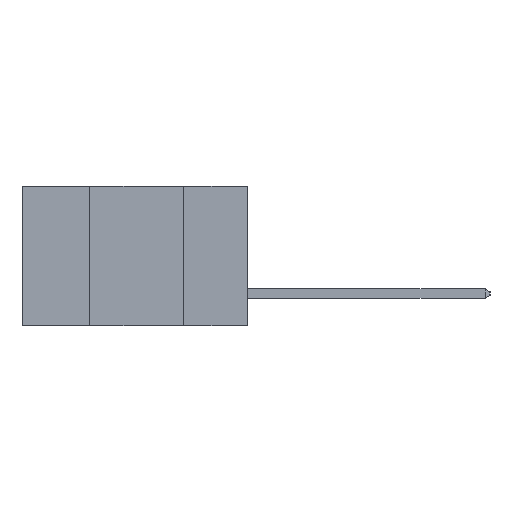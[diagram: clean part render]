
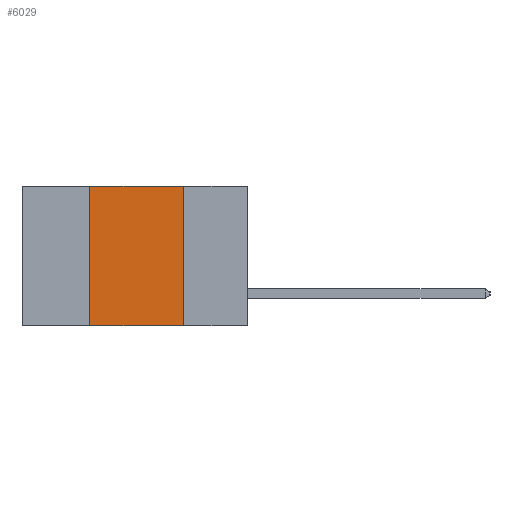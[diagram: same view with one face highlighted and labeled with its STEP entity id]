
A CAD part, left-side view. The second image highlights one B-rep face of the part: STEP entity #6029.
In plain terms, the highlighted planar face has unit normal (-1, 0, 0).
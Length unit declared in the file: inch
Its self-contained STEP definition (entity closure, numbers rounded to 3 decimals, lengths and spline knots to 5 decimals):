
#558 = EDGE_CURVE ( 'NONE', #3124, #1800, #10433, .T. ) ;
#740 = PLANE ( 'NONE',  #9069 ) ;
#755 = VECTOR ( 'NONE', #6571, 39.37008 ) ;
#814 = CARTESIAN_POINT ( 'NONE',  ( 0., 0.42, 0. ) ) ;
#1522 = CARTESIAN_POINT ( 'NONE',  ( 0., 0.17, 0. ) ) ;
#1800 = VERTEX_POINT ( 'NONE', #1522 ) ;
#2483 = DIRECTION ( 'NONE',  ( 0., 0., -1. ) ) ;
#2493 = DIRECTION ( 'NONE',  ( 1., 0., 0. ) ) ;
#3045 = VERTEX_POINT ( 'NONE', #4109 ) ;
#3124 = VERTEX_POINT ( 'NONE', #10151 ) ;
#3153 = VECTOR ( 'NONE', #2483, 39.37008 ) ;
#3307 = ORIENTED_EDGE ( 'NONE', *, *, #558, .F. ) ;
#3781 = EDGE_LOOP ( 'NONE', ( #4730, #3307, #5022, #6675 ) ) ;
#4109 = CARTESIAN_POINT ( 'NONE',  ( 0., 0.17, -0.37 ) ) ;
#4523 = VECTOR ( 'NONE', #8162, 39.37008 ) ;
#4583 = VECTOR ( 'NONE', #8148, 39.37008 ) ;
#4730 = ORIENTED_EDGE ( 'NONE', *, *, #8755, .F. ) ;
#4865 = CARTESIAN_POINT ( 'NONE',  ( 0., 0.42, -0.37 ) ) ;
#5022 = ORIENTED_EDGE ( 'NONE', *, *, #8813, .F. ) ;
#5460 = LINE ( 'NONE', #8140, #755 ) ;
#6029 = ADVANCED_FACE ( 'NONE', ( #8619 ), #740, .F. ) ;
#6571 = DIRECTION ( 'NONE',  ( 0., -1., 0. ) ) ;
#6675 = ORIENTED_EDGE ( 'NONE', *, *, #7267, .T. ) ;
#7267 = EDGE_CURVE ( 'NONE', #8695, #3045, #5460, .T. ) ;
#8058 = CARTESIAN_POINT ( 'NONE',  ( 0., 0.6, 0. ) ) ;
#8090 = DIRECTION ( 'NONE',  ( 0., 0., -1. ) ) ;
#8140 = CARTESIAN_POINT ( 'NONE',  ( 0., 0.6, -0.37 ) ) ;
#8148 = DIRECTION ( 'NONE',  ( 0., 0., 1. ) ) ;
#8162 = DIRECTION ( 'NONE',  ( 0., -1., 0. ) ) ;
#8619 = FACE_OUTER_BOUND ( 'NONE', #3781, .T. ) ;
#8695 = VERTEX_POINT ( 'NONE', #4865 ) ;
#8755 = EDGE_CURVE ( 'NONE', #1800, #3045, #9632, .T. ) ;
#8778 = CARTESIAN_POINT ( 'NONE',  ( 0., 0.17, 0. ) ) ;
#8813 = EDGE_CURVE ( 'NONE', #8695, #3124, #8918, .T. ) ;
#8918 = LINE ( 'NONE', #814, #4583 ) ;
#9005 = CARTESIAN_POINT ( 'NONE',  ( 0., 0.6, 0. ) ) ;
#9069 = AXIS2_PLACEMENT_3D ( 'NONE', #8058, #2493, #8090 ) ;
#9632 = LINE ( 'NONE', #8778, #3153 ) ;
#10151 = CARTESIAN_POINT ( 'NONE',  ( 0., 0.42, 0. ) ) ;
#10433 = LINE ( 'NONE', #9005, #4523 ) ;
